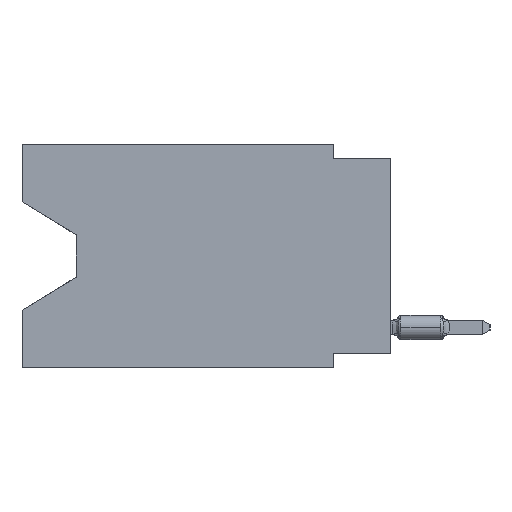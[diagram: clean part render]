
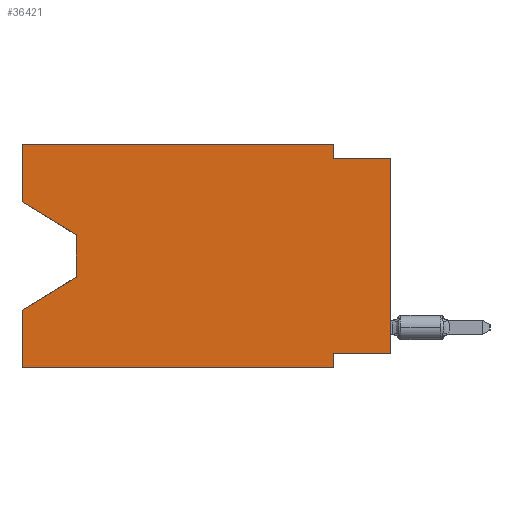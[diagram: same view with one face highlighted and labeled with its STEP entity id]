
A CAD part, left-side view. The second image highlights one B-rep face of the part: STEP entity #36421.
In plain terms, the highlighted planar face has unit normal (-1, 0, 0).
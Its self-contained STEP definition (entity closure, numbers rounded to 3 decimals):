
#527 = ORIENTED_EDGE ( 'NONE', *, *, #19538, .T. ) ;
#1397 = CARTESIAN_POINT ( 'NONE',  ( 0., 2.54, 0. ) ) ;
#1562 = VERTEX_POINT ( 'NONE', #10217 ) ;
#1594 = VERTEX_POINT ( 'NONE', #14372 ) ;
#1691 = LINE ( 'NONE', #22720, #37277 ) ;
#1891 = VECTOR ( 'NONE', #20567, 1000. ) ;
#1965 = VECTOR ( 'NONE', #18006, 1000. ) ;
#3506 = VERTEX_POINT ( 'NONE', #44763 ) ;
#3912 = CARTESIAN_POINT ( 'NONE',  ( 0., 13.97, -5.893 ) ) ;
#4046 = CARTESIAN_POINT ( 'NONE',  ( 0., 2.54, 0. ) ) ;
#4640 = FACE_OUTER_BOUND ( 'NONE', #9305, .T. ) ;
#4664 = LINE ( 'NONE', #34883, #1891 ) ;
#4763 = DIRECTION ( 'NONE',  ( 0., 0., -1. ) ) ;
#5466 = EDGE_CURVE ( 'NONE', #1562, #12287, #20799, .T. ) ;
#5556 = DIRECTION ( 'NONE',  ( 0., 1., 0. ) ) ;
#6024 = LINE ( 'NONE', #1397, #19734 ) ;
#6226 = ORIENTED_EDGE ( 'NONE', *, *, #18500, .T. ) ;
#6264 = ORIENTED_EDGE ( 'NONE', *, *, #5466, .T. ) ;
#6915 = LINE ( 'NONE', #3912, #1965 ) ;
#8094 = VERTEX_POINT ( 'NONE', #4046 ) ;
#8925 = VERTEX_POINT ( 'NONE', #42027 ) ;
#9269 = VECTOR ( 'NONE', #37938, 1000. ) ;
#9305 = EDGE_LOOP ( 'NONE', ( #527, #13319, #30563, #20948, #6264, #19455, #27658, #6226, #16560, #10008, #24115, #16874 ) ) ;
#9704 = EDGE_CURVE ( 'NONE', #38599, #8094, #1691, .T. ) ;
#10008 = ORIENTED_EDGE ( 'NONE', *, *, #11045, .F. ) ;
#10124 = EDGE_CURVE ( 'NONE', #1594, #38599, #4664, .T. ) ;
#10217 = CARTESIAN_POINT ( 'NONE',  ( 0., 16.383, -9.906 ) ) ;
#10453 = VECTOR ( 'NONE', #39034, 1000. ) ;
#11045 = EDGE_CURVE ( 'NONE', #8094, #8925, #6024, .T. ) ;
#11094 = EDGE_CURVE ( 'NONE', #24174, #26526, #40200, .T. ) ;
#11998 = DIRECTION ( 'NONE',  ( 0., 0., 1. ) ) ;
#12287 = VERTEX_POINT ( 'NONE', #16639 ) ;
#12719 = CARTESIAN_POINT ( 'NONE',  ( 0., 16.383, -7.36 ) ) ;
#13319 = ORIENTED_EDGE ( 'NONE', *, *, #35574, .T. ) ;
#14372 = CARTESIAN_POINT ( 'NONE',  ( 0., 16.383, -2.546 ) ) ;
#14624 = VERTEX_POINT ( 'NONE', #12719 ) ;
#14848 = LINE ( 'NONE', #25485, #34167 ) ;
#15584 = CARTESIAN_POINT ( 'NONE',  ( 0., 13.97, -4.013 ) ) ;
#15778 = DIRECTION ( 'NONE',  ( 0., -1., 0. ) ) ;
#16560 = ORIENTED_EDGE ( 'NONE', *, *, #33245, .F. ) ;
#16639 = CARTESIAN_POINT ( 'NONE',  ( 0., 2.54, -9.906 ) ) ;
#16671 = LINE ( 'NONE', #42055, #9269 ) ;
#16874 = ORIENTED_EDGE ( 'NONE', *, *, #10124, .F. ) ;
#18006 = DIRECTION ( 'NONE',  ( 0., 0.855, -0.519 ) ) ;
#18500 = EDGE_CURVE ( 'NONE', #24174, #43789, #37190, .T. ) ;
#19455 = ORIENTED_EDGE ( 'NONE', *, *, #30539, .F. ) ;
#19538 = EDGE_CURVE ( 'NONE', #1594, #19670, #16671, .T. ) ;
#19670 = VERTEX_POINT ( 'NONE', #32354 ) ;
#19734 = VECTOR ( 'NONE', #33052, 1000. ) ;
#20303 = DIRECTION ( 'NONE',  ( 0., 0., 1. ) ) ;
#20567 = DIRECTION ( 'NONE',  ( 0., 0., 1. ) ) ;
#20799 = LINE ( 'NONE', #28645, #10453 ) ;
#20945 = VECTOR ( 'NONE', #24734, 1000. ) ;
#20948 = ORIENTED_EDGE ( 'NONE', *, *, #42700, .F. ) ;
#22172 = CARTESIAN_POINT ( 'NONE',  ( 0., 0., -0.635 ) ) ;
#22429 = CARTESIAN_POINT ( 'NONE',  ( 0., 16.383, 0. ) ) ;
#22657 = CARTESIAN_POINT ( 'NONE',  ( 0., 0., -9.271 ) ) ;
#22720 = CARTESIAN_POINT ( 'NONE',  ( 0., 16.383, 0. ) ) ;
#23298 = LINE ( 'NONE', #27225, #38369 ) ;
#24115 = ORIENTED_EDGE ( 'NONE', *, *, #9704, .F. ) ;
#24174 = VERTEX_POINT ( 'NONE', #44212 ) ;
#24734 = DIRECTION ( 'NONE',  ( 0., -1., 0. ) ) ;
#24791 = VECTOR ( 'NONE', #4763, 1000. ) ;
#25485 = CARTESIAN_POINT ( 'NONE',  ( 0., 2.54, -9.906 ) ) ;
#25643 = PLANE ( 'NONE',  #26265 ) ;
#26265 = AXIS2_PLACEMENT_3D ( 'NONE', #22429, #36948, #39519 ) ;
#26526 = VERTEX_POINT ( 'NONE', #44666 ) ;
#27225 = CARTESIAN_POINT ( 'NONE',  ( 0., 16.383, 0. ) ) ;
#27658 = ORIENTED_EDGE ( 'NONE', *, *, #11094, .F. ) ;
#28645 = CARTESIAN_POINT ( 'NONE',  ( 0., 16.383, -9.906 ) ) ;
#30539 = EDGE_CURVE ( 'NONE', #26526, #12287, #14848, .T. ) ;
#30563 = ORIENTED_EDGE ( 'NONE', *, *, #36721, .T. ) ;
#31948 = VECTOR ( 'NONE', #11998, 1000. ) ;
#32354 = CARTESIAN_POINT ( 'NONE',  ( 0., 13.97, -4.013 ) ) ;
#33052 = DIRECTION ( 'NONE',  ( 0., 0., -1. ) ) ;
#33245 = EDGE_CURVE ( 'NONE', #8925, #43789, #35136, .T. ) ;
#33744 = VECTOR ( 'NONE', #5556, 1000. ) ;
#34167 = VECTOR ( 'NONE', #39583, 1000. ) ;
#34883 = CARTESIAN_POINT ( 'NONE',  ( 0., 16.383, 0. ) ) ;
#35136 = LINE ( 'NONE', #41612, #20945 ) ;
#35574 = EDGE_CURVE ( 'NONE', #19670, #3506, #37303, .T. ) ;
#36421 = ADVANCED_FACE ( 'NONE', ( #4640 ), #25643, .F. ) ;
#36721 = EDGE_CURVE ( 'NONE', #3506, #14624, #6915, .T. ) ;
#36948 = DIRECTION ( 'NONE',  ( 1., 0., 0. ) ) ;
#37190 = LINE ( 'NONE', #43649, #31948 ) ;
#37277 = VECTOR ( 'NONE', #15778, 1000. ) ;
#37303 = LINE ( 'NONE', #15584, #24791 ) ;
#37938 = DIRECTION ( 'NONE',  ( 0., -0.855, -0.519 ) ) ;
#38369 = VECTOR ( 'NONE', #20303, 1000. ) ;
#38599 = VERTEX_POINT ( 'NONE', #44228 ) ;
#39034 = DIRECTION ( 'NONE',  ( 0., -1., 0. ) ) ;
#39519 = DIRECTION ( 'NONE',  ( 0., 0., -1. ) ) ;
#39583 = DIRECTION ( 'NONE',  ( 0., 0., -1. ) ) ;
#40200 = LINE ( 'NONE', #22657, #33744 ) ;
#41612 = CARTESIAN_POINT ( 'NONE',  ( 0., 0., -0.635 ) ) ;
#42027 = CARTESIAN_POINT ( 'NONE',  ( 0., 2.54, -0.635 ) ) ;
#42055 = CARTESIAN_POINT ( 'NONE',  ( 0., 16.383, -2.546 ) ) ;
#42700 = EDGE_CURVE ( 'NONE', #1562, #14624, #23298, .T. ) ;
#43649 = CARTESIAN_POINT ( 'NONE',  ( 0., 0., 0. ) ) ;
#43789 = VERTEX_POINT ( 'NONE', #22172 ) ;
#44212 = CARTESIAN_POINT ( 'NONE',  ( 0., 0., -9.271 ) ) ;
#44228 = CARTESIAN_POINT ( 'NONE',  ( 0., 16.383, 0. ) ) ;
#44666 = CARTESIAN_POINT ( 'NONE',  ( 0., 2.54, -9.271 ) ) ;
#44763 = CARTESIAN_POINT ( 'NONE',  ( 0., 13.97, -5.893 ) ) ;
